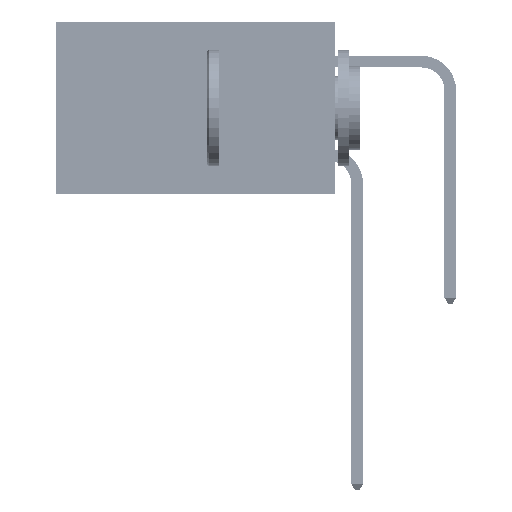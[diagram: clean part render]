
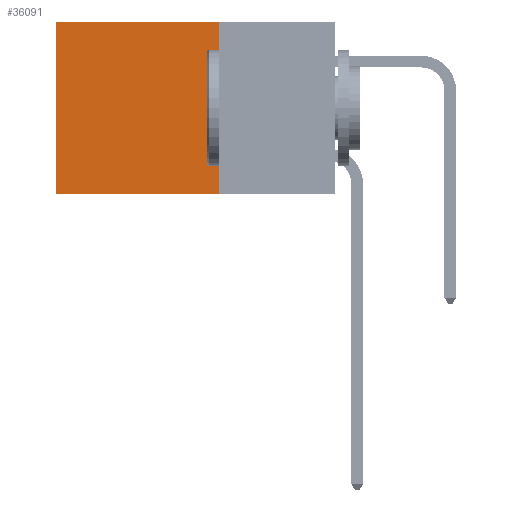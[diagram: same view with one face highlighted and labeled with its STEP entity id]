
A CAD part, left-side view. The second image highlights one B-rep face of the part: STEP entity #36091.
In plain terms, the highlighted planar face has unit normal (-1, 0, 0).
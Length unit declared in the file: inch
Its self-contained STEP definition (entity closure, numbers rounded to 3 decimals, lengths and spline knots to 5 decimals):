
#1126 = VERTEX_POINT ( 'NONE', #40922 ) ;
#2033 = CARTESIAN_POINT ( 'NONE',  ( 0.2875, 0.6, 0. ) ) ;
#6053 = DIRECTION ( 'NONE',  ( 0., 1., 0. ) ) ;
#6076 = VECTOR ( 'NONE', #30010, 39.37008 ) ;
#6293 = CARTESIAN_POINT ( 'NONE',  ( 0.2875, 0.6, 0. ) ) ;
#7032 = VECTOR ( 'NONE', #6053, 39.37008 ) ;
#8630 = LINE ( 'NONE', #38023, #6076 ) ;
#9177 = ORIENTED_EDGE ( 'NONE', *, *, #27749, .F. ) ;
#10132 = CARTESIAN_POINT ( 'NONE',  ( 0.2875, 0.25, 0. ) ) ;
#10396 = DIRECTION ( 'NONE',  ( 0., 0., -1. ) ) ;
#12129 = VECTOR ( 'NONE', #10396, 39.37008 ) ;
#19356 = VERTEX_POINT ( 'NONE', #33733 ) ;
#23291 = DIRECTION ( 'NONE',  ( 1., 0., 0. ) ) ;
#24941 = EDGE_CURVE ( 'NONE', #1126, #45047, #8630, .T. ) ;
#25034 = DIRECTION ( 'NONE',  ( 0., 0., -1. ) ) ;
#26326 = ORIENTED_EDGE ( 'NONE', *, *, #47370, .T. ) ;
#27749 = EDGE_CURVE ( 'NONE', #19356, #1126, #45316, .T. ) ;
#27760 = ORIENTED_EDGE ( 'NONE', *, *, #27991, .T. ) ;
#27991 = EDGE_CURVE ( 'NONE', #34460, #45047, #45938, .T. ) ;
#30010 = DIRECTION ( 'NONE',  ( 0., 1., 0. ) ) ;
#30753 = FACE_OUTER_BOUND ( 'NONE', #42146, .T. ) ;
#33733 = CARTESIAN_POINT ( 'NONE',  ( 0.2875, 0.25, 0. ) ) ;
#34460 = VERTEX_POINT ( 'NONE', #2033 ) ;
#36091 = ADVANCED_FACE ( 'NONE', ( #30753 ), #43614, .F. ) ;
#38023 = CARTESIAN_POINT ( 'NONE',  ( 0.2875, 0.25, -0.37 ) ) ;
#40824 = AXIS2_PLACEMENT_3D ( 'NONE', #47756, #23291, #51847 ) ;
#40827 = LINE ( 'NONE', #10132, #7032 ) ;
#40922 = CARTESIAN_POINT ( 'NONE',  ( 0.2875, 0.25, -0.37 ) ) ;
#42146 = EDGE_LOOP ( 'NONE', ( #27760, #42904, #9177, #26326 ) ) ;
#42904 = ORIENTED_EDGE ( 'NONE', *, *, #24941, .F. ) ;
#43614 = PLANE ( 'NONE',  #40824 ) ;
#44028 = VECTOR ( 'NONE', #25034, 39.37008 ) ;
#45047 = VERTEX_POINT ( 'NONE', #50839 ) ;
#45316 = LINE ( 'NONE', #45548, #44028 ) ;
#45548 = CARTESIAN_POINT ( 'NONE',  ( 0.2875, 0.25, 0. ) ) ;
#45938 = LINE ( 'NONE', #6293, #12129 ) ;
#47370 = EDGE_CURVE ( 'NONE', #19356, #34460, #40827, .T. ) ;
#47756 = CARTESIAN_POINT ( 'NONE',  ( 0.2875, 0.25, 0. ) ) ;
#50839 = CARTESIAN_POINT ( 'NONE',  ( 0.2875, 0.6, -0.37 ) ) ;
#51847 = DIRECTION ( 'NONE',  ( 0., 0., -1. ) ) ;
